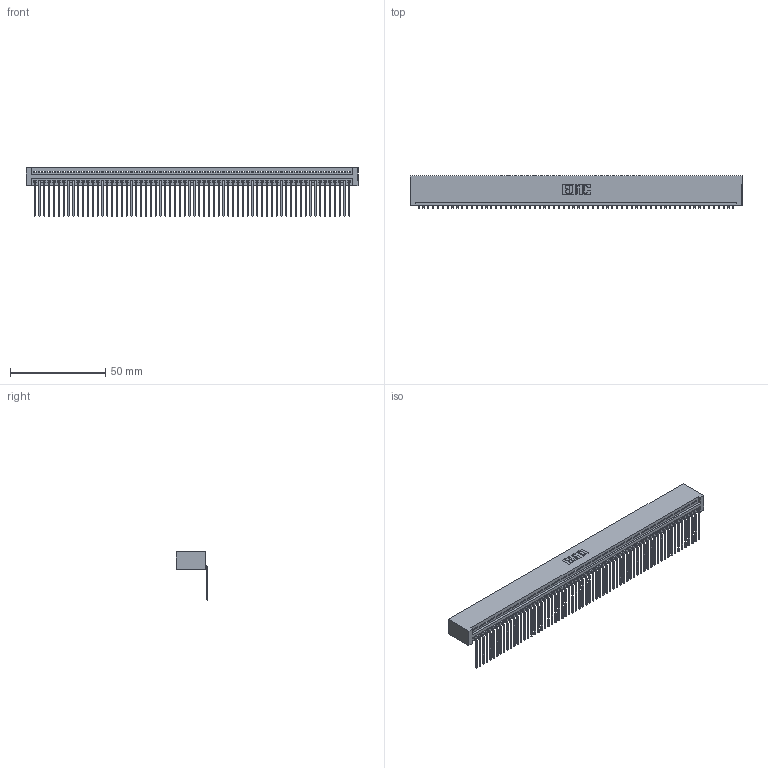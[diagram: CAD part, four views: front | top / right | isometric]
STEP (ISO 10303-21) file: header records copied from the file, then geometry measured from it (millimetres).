
FILE_DESCRIPTION (( 'STEP AP203' ), '1' );
FILE_NAME ('345-066-559-101.STEP', '2018-09-29T00:18:14', ( '' ), ( '' ), 'SwSTEP 2.0', 'SolidWorks 2016', '' );
FILE_SCHEMA (( 'CONFIG_CONTROL_DESIGN' ));
Length unit declared in the file: inch
Products named in the file (3): 345-066-559-101; 345 Part_No Mounting Lugs; 345-292-001_558 559 Tail - 1
Assembly tree (67 placements, depth 2):
  345-066-559-101
    345 Part_No Mounting Lugs
    345-292-001_558 559 Tail - 1  x66
Bounding box: 174.24 x 16.75 x 25.53 mm (x, y, z)
Volume: 17550.7 mm3; surface area: 25131.8 mm2
Topology: 67 solids, 67 shells, 4078 faces, 12329 edges, 8130 vertices
Faces by surface type: plane 2848, cylinder 1230
Entity records: 46249 total; most frequent: ORIENTED_EDGE 8018, CARTESIAN_POINT 8018, DIRECTION 6961, EDGE_CURVE 4009, LINE 3621, VECTOR 3621, VERTEX_POINT 2670, AXIS2_PLACEMENT_3D 1670
